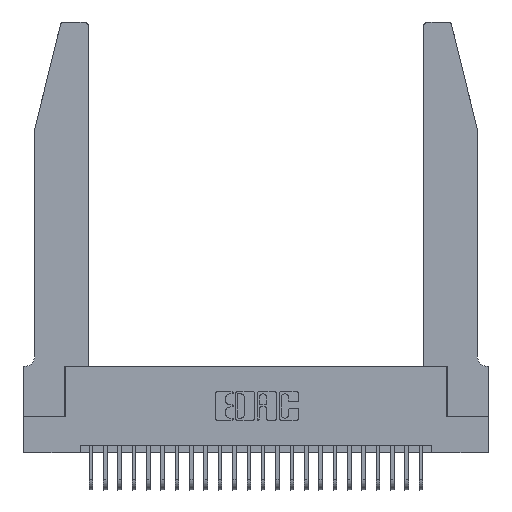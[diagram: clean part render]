
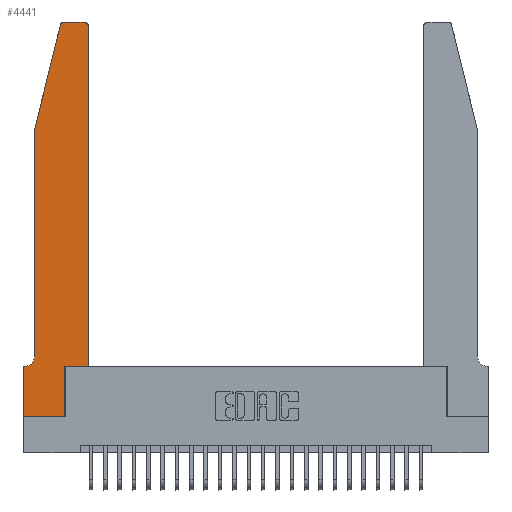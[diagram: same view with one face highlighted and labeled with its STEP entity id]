
A CAD part, top view. The second image highlights one B-rep face of the part: STEP entity #4441.
In plain terms, the highlighted planar face has unit normal (0, 0, 1).
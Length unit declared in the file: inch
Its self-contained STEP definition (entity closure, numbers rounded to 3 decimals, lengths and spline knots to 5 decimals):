
#118 = CARTESIAN_POINT ( 'NONE',  ( 0.2865, 0., 0.37 ) ) ;
#254 = LINE ( 'NONE', #10254, #21749 ) ;
#387 = VERTEX_POINT ( 'NONE', #19968 ) ;
#734 = VERTEX_POINT ( 'NONE', #4361 ) ;
#980 = CARTESIAN_POINT ( 'NONE',  ( 0.4505, 0.35, 0.37 ) ) ;
#1202 = VECTOR ( 'NONE', #2515, 39.37008 ) ;
#1545 = EDGE_CURVE ( 'NONE', #16911, #24357, #7369, .T. ) ;
#1565 = DIRECTION ( 'NONE',  ( 1., 0., 0. ) ) ;
#2249 = VECTOR ( 'NONE', #11698, 39.37008 ) ;
#2333 = AXIS2_PLACEMENT_3D ( 'NONE', #13565, #15678, #2826 ) ;
#2515 = DIRECTION ( 'NONE',  ( 1., 0., 0. ) ) ;
#2600 = CIRCLE ( 'NONE', #14317, 0.03 ) ;
#2637 = ORIENTED_EDGE ( 'NONE', *, *, #12291, .T. ) ;
#2826 = DIRECTION ( 'NONE',  ( 1., 0., 0. ) ) ;
#3159 = CARTESIAN_POINT ( 'NONE',  ( 0.0755, 2., 0.37 ) ) ;
#3164 = DIRECTION ( 'NONE',  ( 0., 1., 0. ) ) ;
#3228 = EDGE_CURVE ( 'NONE', #22403, #21755, #11939, .T. ) ;
#3678 = ORIENTED_EDGE ( 'NONE', *, *, #22922, .T. ) ;
#4361 = CARTESIAN_POINT ( 'NONE',  ( 0.25487, 2.72718, 0.37 ) ) ;
#4441 = ADVANCED_FACE ( 'NONE', ( #27446 ), #26204, .T. ) ;
#4750 = EDGE_CURVE ( 'NONE', #23168, #26682, #25322, .T. ) ;
#5065 = LINE ( 'NONE', #980, #10154 ) ;
#5166 = CARTESIAN_POINT ( 'NONE',  ( 0.0755, 0.35, 0.37 ) ) ;
#5213 = VERTEX_POINT ( 'NONE', #18127 ) ;
#5339 = DIRECTION ( 'NONE',  ( 0., 0., -1. ) ) ;
#5372 = CARTESIAN_POINT ( 'NONE',  ( 0.2865, 0.35, 0.37 ) ) ;
#5549 = CARTESIAN_POINT ( 'NONE',  ( 0.0055, 0.35, 0.37 ) ) ;
#5802 = CARTESIAN_POINT ( 'NONE',  ( 0.0755, 0.42, 0.37 ) ) ;
#6005 = VECTOR ( 'NONE', #10355, 39.37008 ) ;
#6185 = ORIENTED_EDGE ( 'NONE', *, *, #23274, .T. ) ;
#7369 = LINE ( 'NONE', #25137, #6005 ) ;
#8644 = ORIENTED_EDGE ( 'NONE', *, *, #22715, .T. ) ;
#8678 = ORIENTED_EDGE ( 'NONE', *, *, #24481, .T. ) ;
#9358 = ORIENTED_EDGE ( 'NONE', *, *, #13274, .T. ) ;
#10154 = VECTOR ( 'NONE', #3164, 39.37008 ) ;
#10213 = EDGE_CURVE ( 'NONE', #21755, #10781, #17436, .T. ) ;
#10254 = CARTESIAN_POINT ( 'NONE',  ( 0.0755, 2., 0.37 ) ) ;
#10355 = DIRECTION ( 'NONE',  ( 1., 0., 0. ) ) ;
#10781 = VERTEX_POINT ( 'NONE', #25942 ) ;
#11152 = CARTESIAN_POINT ( 'NONE',  ( 0.284, 2.72, 0.37 ) ) ;
#11372 = LINE ( 'NONE', #19635, #1202 ) ;
#11575 = CARTESIAN_POINT ( 'NONE',  ( 0.4205, 2.75, 0.37 ) ) ;
#11698 = DIRECTION ( 'NONE',  ( -1., 0., 0. ) ) ;
#11786 = ORIENTED_EDGE ( 'NONE', *, *, #4750, .T. ) ;
#11939 = CIRCLE ( 'NONE', #20248, 0.07 ) ;
#12291 = EDGE_CURVE ( 'NONE', #10781, #14776, #27045, .T. ) ;
#12364 = DIRECTION ( 'NONE',  ( 0., -1., 0. ) ) ;
#13189 = CARTESIAN_POINT ( 'NONE',  ( 0., 0., 0.37 ) ) ;
#13274 = EDGE_CURVE ( 'NONE', #24357, #23168, #5065, .T. ) ;
#13293 = DIRECTION ( 'NONE',  ( 1., 0., 0. ) ) ;
#13565 = CARTESIAN_POINT ( 'NONE',  ( 0., 0.35, 0.37 ) ) ;
#14256 = VERTEX_POINT ( 'NONE', #118 ) ;
#14317 = AXIS2_PLACEMENT_3D ( 'NONE', #11152, #25923, #13293 ) ;
#14358 = DIRECTION ( 'NONE',  ( 0., 1., 0. ) ) ;
#14476 = DIRECTION ( 'NONE',  ( 0., 0., 1. ) ) ;
#14776 = VERTEX_POINT ( 'NONE', #13189 ) ;
#14836 = CARTESIAN_POINT ( 'NONE',  ( 0.4505, 2.72, 0.37 ) ) ;
#15324 = EDGE_LOOP ( 'NONE', ( #3678, #8644, #23972, #22488, #24301, #24133, #2637, #6185, #8678, #22858, #9358, #11786 ) ) ;
#15678 = DIRECTION ( 'NONE',  ( 0., 0., 1. ) ) ;
#15814 = VECTOR ( 'NONE', #20625, 39.37008 ) ;
#15908 = DIRECTION ( 'NONE',  ( -0.239, -0.971, 0. ) ) ;
#16360 = CARTESIAN_POINT ( 'NONE',  ( 0.2865, 0.35, 0.37 ) ) ;
#16500 = VECTOR ( 'NONE', #14358, 39.37008 ) ;
#16911 = VERTEX_POINT ( 'NONE', #5372 ) ;
#17436 = LINE ( 'NONE', #5166, #22419 ) ;
#17931 = DIRECTION ( 'NONE',  ( -1., 0., 0. ) ) ;
#18105 = CARTESIAN_POINT ( 'NONE',  ( 0.0055, 0.42, 0.37 ) ) ;
#18127 = CARTESIAN_POINT ( 'NONE',  ( 0.284, 2.75, 0.37 ) ) ;
#19635 = CARTESIAN_POINT ( 'NONE',  ( 0., 0., 0.37 ) ) ;
#19968 = CARTESIAN_POINT ( 'NONE',  ( 0.0755, 2., 0.37 ) ) ;
#20206 = CARTESIAN_POINT ( 'NONE',  ( 0.2605, 2.75, 0.37 ) ) ;
#20248 = AXIS2_PLACEMENT_3D ( 'NONE', #18105, #5339, #20253 ) ;
#20253 = DIRECTION ( 'NONE',  ( -1., 0., 0. ) ) ;
#20365 = LINE ( 'NONE', #3159, #25310 ) ;
#20625 = DIRECTION ( 'NONE',  ( 0., -1., 0. ) ) ;
#21749 = VECTOR ( 'NONE', #12364, 39.37008 ) ;
#21755 = VERTEX_POINT ( 'NONE', #5549 ) ;
#22403 = VERTEX_POINT ( 'NONE', #5802 ) ;
#22419 = VECTOR ( 'NONE', #17931, 39.37008 ) ;
#22488 = ORIENTED_EDGE ( 'NONE', *, *, #25647, .T. ) ;
#22715 = EDGE_CURVE ( 'NONE', #5213, #734, #2600, .T. ) ;
#22755 = CARTESIAN_POINT ( 'NONE',  ( 0., 0., 0.37 ) ) ;
#22821 = LINE ( 'NONE', #16360, #16500 ) ;
#22858 = ORIENTED_EDGE ( 'NONE', *, *, #1545, .T. ) ;
#22922 = EDGE_CURVE ( 'NONE', #26682, #5213, #24949, .T. ) ;
#23168 = VERTEX_POINT ( 'NONE', #14836 ) ;
#23274 = EDGE_CURVE ( 'NONE', #14776, #14256, #11372, .T. ) ;
#23972 = ORIENTED_EDGE ( 'NONE', *, *, #27639, .T. ) ;
#24133 = ORIENTED_EDGE ( 'NONE', *, *, #10213, .T. ) ;
#24301 = ORIENTED_EDGE ( 'NONE', *, *, #3228, .T. ) ;
#24357 = VERTEX_POINT ( 'NONE', #26445 ) ;
#24481 = EDGE_CURVE ( 'NONE', #14256, #16911, #22821, .T. ) ;
#24949 = LINE ( 'NONE', #20206, #2249 ) ;
#25137 = CARTESIAN_POINT ( 'NONE',  ( 0.4505, 0.35, 0.37 ) ) ;
#25207 = AXIS2_PLACEMENT_3D ( 'NONE', #27106, #14476, #1565 ) ;
#25310 = VECTOR ( 'NONE', #15908, 39.37008 ) ;
#25322 = CIRCLE ( 'NONE', #25207, 0.03 ) ;
#25647 = EDGE_CURVE ( 'NONE', #387, #22403, #254, .T. ) ;
#25923 = DIRECTION ( 'NONE',  ( 0., 0., 1. ) ) ;
#25942 = CARTESIAN_POINT ( 'NONE',  ( 0., 0.35, 0.37 ) ) ;
#26204 = PLANE ( 'NONE',  #2333 ) ;
#26445 = CARTESIAN_POINT ( 'NONE',  ( 0.4505, 0.35, 0.37 ) ) ;
#26682 = VERTEX_POINT ( 'NONE', #11575 ) ;
#27045 = LINE ( 'NONE', #22755, #15814 ) ;
#27106 = CARTESIAN_POINT ( 'NONE',  ( 0.4205, 2.72, 0.37 ) ) ;
#27446 = FACE_OUTER_BOUND ( 'NONE', #15324, .T. ) ;
#27639 = EDGE_CURVE ( 'NONE', #734, #387, #20365, .T. ) ;
